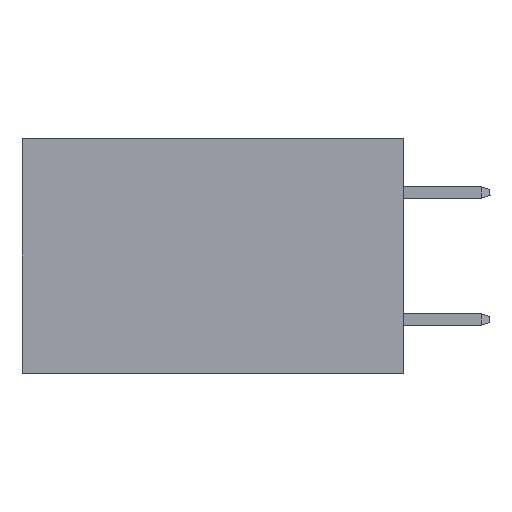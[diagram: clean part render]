
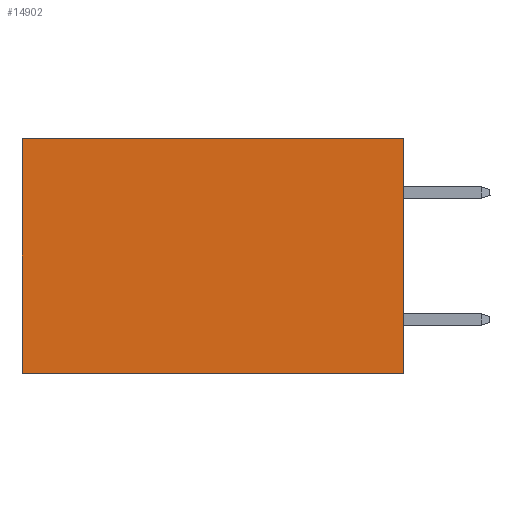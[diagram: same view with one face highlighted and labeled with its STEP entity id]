
A CAD part, left-side view. The second image highlights one B-rep face of the part: STEP entity #14902.
In plain terms, the highlighted planar face has unit normal (-1, 0, 0).
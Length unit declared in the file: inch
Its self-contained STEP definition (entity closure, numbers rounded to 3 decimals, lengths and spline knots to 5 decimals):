
#3066 = LINE ( 'NONE', #27603, #24082 ) ;
#5937 = ORIENTED_EDGE ( 'NONE', *, *, #27309, .F. ) ;
#6300 = ORIENTED_EDGE ( 'NONE', *, *, #30004, .F. ) ;
#7146 = AXIS2_PLACEMENT_3D ( 'NONE', #40788, #20078, #33591 ) ;
#7615 = ORIENTED_EDGE ( 'NONE', *, *, #42618, .T. ) ;
#9552 = VERTEX_POINT ( 'NONE', #40141 ) ;
#9654 = EDGE_LOOP ( 'NONE', ( #7615, #5937, #6300, #43131 ) ) ;
#11266 = DIRECTION ( 'NONE',  ( 0., 1., 0. ) ) ;
#11477 = LINE ( 'NONE', #18473, #29132 ) ;
#12048 = CARTESIAN_POINT ( 'NONE',  ( 0.2875, 0., -0.37 ) ) ;
#13300 = PLANE ( 'NONE',  #7146 ) ;
#14054 = CARTESIAN_POINT ( 'NONE',  ( 0.2875, 0.6, 0. ) ) ;
#14902 = ADVANCED_FACE ( 'NONE', ( #23464 ), #13300, .F. ) ;
#15545 = VECTOR ( 'NONE', #39434, 39.37008 ) ;
#16079 = CARTESIAN_POINT ( 'NONE',  ( 0.2875, 0., -0.37 ) ) ;
#17271 = DIRECTION ( 'NONE',  ( 0., 0., -1. ) ) ;
#18473 = CARTESIAN_POINT ( 'NONE',  ( 0.2875, 0., 0. ) ) ;
#19087 = VECTOR ( 'NONE', #29363, 39.37008 ) ;
#19619 = VERTEX_POINT ( 'NONE', #12048 ) ;
#20078 = DIRECTION ( 'NONE',  ( 1., 0., 0. ) ) ;
#22769 = LINE ( 'NONE', #29296, #15545 ) ;
#23464 = FACE_OUTER_BOUND ( 'NONE', #9654, .T. ) ;
#23789 = VERTEX_POINT ( 'NONE', #36652 ) ;
#24082 = VECTOR ( 'NONE', #17271, 39.37008 ) ;
#27309 = EDGE_CURVE ( 'NONE', #19619, #9552, #29139, .T. ) ;
#27603 = CARTESIAN_POINT ( 'NONE',  ( 0.2875, 0.6, 0. ) ) ;
#27960 = VERTEX_POINT ( 'NONE', #14054 ) ;
#29132 = VECTOR ( 'NONE', #11266, 39.37008 ) ;
#29139 = LINE ( 'NONE', #16079, #19087 ) ;
#29296 = CARTESIAN_POINT ( 'NONE',  ( 0.2875, 0., 0. ) ) ;
#29363 = DIRECTION ( 'NONE',  ( 0., 1., 0. ) ) ;
#30004 = EDGE_CURVE ( 'NONE', #23789, #19619, #22769, .T. ) ;
#33591 = DIRECTION ( 'NONE',  ( 0., 0., -1. ) ) ;
#36652 = CARTESIAN_POINT ( 'NONE',  ( 0.2875, 0., 0. ) ) ;
#39434 = DIRECTION ( 'NONE',  ( 0., 0., -1. ) ) ;
#40141 = CARTESIAN_POINT ( 'NONE',  ( 0.2875, 0.6, -0.37 ) ) ;
#40636 = EDGE_CURVE ( 'NONE', #23789, #27960, #11477, .T. ) ;
#40788 = CARTESIAN_POINT ( 'NONE',  ( 0.2875, 0., 0. ) ) ;
#42618 = EDGE_CURVE ( 'NONE', #27960, #9552, #3066, .T. ) ;
#43131 = ORIENTED_EDGE ( 'NONE', *, *, #40636, .T. ) ;
